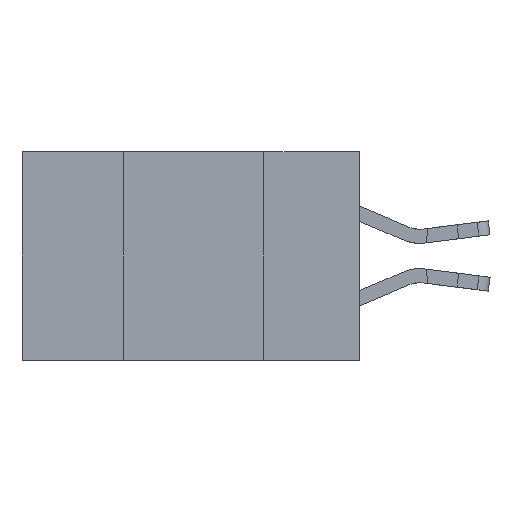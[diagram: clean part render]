
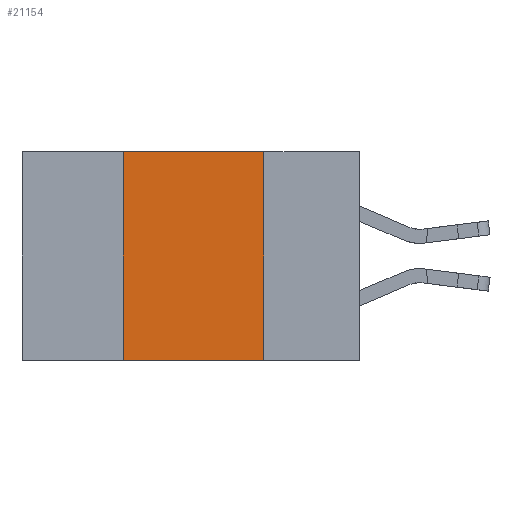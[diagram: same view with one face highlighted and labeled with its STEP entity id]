
A CAD part, left-side view. The second image highlights one B-rep face of the part: STEP entity #21154.
In plain terms, the highlighted planar face has unit normal (-1, 0, 0).
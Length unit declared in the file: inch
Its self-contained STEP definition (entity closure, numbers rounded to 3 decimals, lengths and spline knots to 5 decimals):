
#868 = VERTEX_POINT ( 'NONE', #9648 ) ;
#973 = AXIS2_PLACEMENT_3D ( 'NONE', #19993, #2402, #2293 ) ;
#1546 = VERTEX_POINT ( 'NONE', #4841 ) ;
#2293 = DIRECTION ( 'NONE',  ( 0., 0., -1. ) ) ;
#2402 = DIRECTION ( 'NONE',  ( 1., 0., 0. ) ) ;
#2636 = CARTESIAN_POINT ( 'NONE',  ( 0., 0.42, -0.37 ) ) ;
#3498 = VECTOR ( 'NONE', #29264, 39.37008 ) ;
#3743 = ORIENTED_EDGE ( 'NONE', *, *, #31579, .F. ) ;
#4363 = DIRECTION ( 'NONE',  ( 0., -1., 0. ) ) ;
#4538 = DIRECTION ( 'NONE',  ( 0., 0., 1. ) ) ;
#4610 = CARTESIAN_POINT ( 'NONE',  ( 0., 0.17, 0. ) ) ;
#4841 = CARTESIAN_POINT ( 'NONE',  ( 0., 0.42, 0. ) ) ;
#6652 = VERTEX_POINT ( 'NONE', #2636 ) ;
#9648 = CARTESIAN_POINT ( 'NONE',  ( 0., 0.17, -0.37 ) ) ;
#10069 = LINE ( 'NONE', #4610, #3498 ) ;
#10084 = LINE ( 'NONE', #25064, #31064 ) ;
#10097 = VECTOR ( 'NONE', #4363, 39.37008 ) ;
#11304 = EDGE_LOOP ( 'NONE', ( #19068, #22596, #3743, #16495 ) ) ;
#11828 = CARTESIAN_POINT ( 'NONE',  ( 0., 0.42, 0. ) ) ;
#11857 = FACE_OUTER_BOUND ( 'NONE', #11304, .T. ) ;
#13460 = DIRECTION ( 'NONE',  ( 0., -1., 0. ) ) ;
#16495 = ORIENTED_EDGE ( 'NONE', *, *, #25876, .T. ) ;
#19068 = ORIENTED_EDGE ( 'NONE', *, *, #26540, .F. ) ;
#19268 = CARTESIAN_POINT ( 'NONE',  ( 0., 0.6, -0.37 ) ) ;
#19993 = CARTESIAN_POINT ( 'NONE',  ( 0., 0.6, 0. ) ) ;
#21154 = ADVANCED_FACE ( 'NONE', ( #11857 ), #29541, .F. ) ;
#21235 = CARTESIAN_POINT ( 'NONE',  ( 0., 0.17, 0. ) ) ;
#22596 = ORIENTED_EDGE ( 'NONE', *, *, #30202, .F. ) ;
#22795 = LINE ( 'NONE', #11828, #25942 ) ;
#23320 = LINE ( 'NONE', #19268, #10097 ) ;
#23718 = VERTEX_POINT ( 'NONE', #21235 ) ;
#25064 = CARTESIAN_POINT ( 'NONE',  ( 0., 0.6, 0. ) ) ;
#25876 = EDGE_CURVE ( 'NONE', #6652, #868, #23320, .T. ) ;
#25942 = VECTOR ( 'NONE', #4538, 39.37008 ) ;
#26540 = EDGE_CURVE ( 'NONE', #23718, #868, #10069, .T. ) ;
#29264 = DIRECTION ( 'NONE',  ( 0., 0., -1. ) ) ;
#29541 = PLANE ( 'NONE',  #973 ) ;
#30202 = EDGE_CURVE ( 'NONE', #1546, #23718, #10084, .T. ) ;
#31064 = VECTOR ( 'NONE', #13460, 39.37008 ) ;
#31579 = EDGE_CURVE ( 'NONE', #6652, #1546, #22795, .T. ) ;
